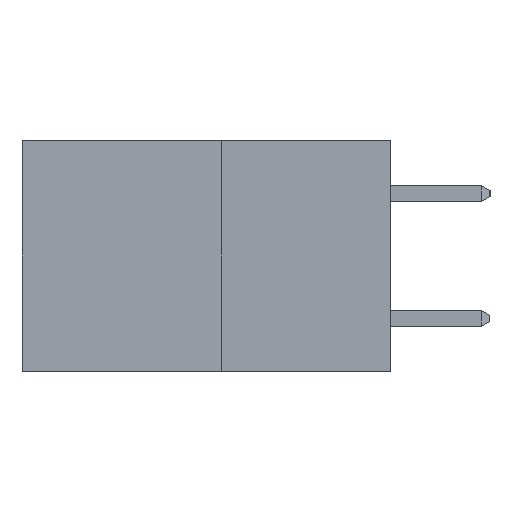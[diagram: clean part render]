
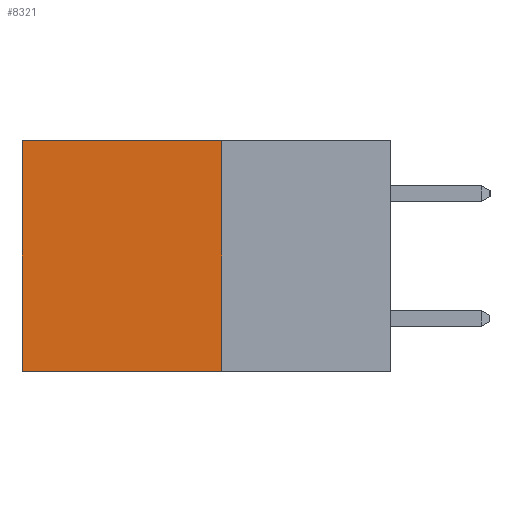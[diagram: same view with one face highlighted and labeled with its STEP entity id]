
A CAD part, left-side view. The second image highlights one B-rep face of the part: STEP entity #8321.
In plain terms, the highlighted planar face has unit normal (-1, 0, 0).
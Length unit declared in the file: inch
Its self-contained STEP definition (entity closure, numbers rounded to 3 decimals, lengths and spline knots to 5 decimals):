
#217 = VECTOR ( 'NONE', #8295, 39.37008 ) ;
#416 = VERTEX_POINT ( 'NONE', #7697 ) ;
#633 = CARTESIAN_POINT ( 'NONE',  ( 0.277, 0.59, -0.37 ) ) ;
#1566 = ORIENTED_EDGE ( 'NONE', *, *, #2854, .T. ) ;
#1673 = DIRECTION ( 'NONE',  ( 0., 0., -1. ) ) ;
#1694 = CARTESIAN_POINT ( 'NONE',  ( 0.277, 0.27, -0.37 ) ) ;
#1730 = VECTOR ( 'NONE', #4963, 39.37008 ) ;
#2251 = ORIENTED_EDGE ( 'NONE', *, *, #8538, .F. ) ;
#2705 = LINE ( 'NONE', #8316, #217 ) ;
#2854 = EDGE_CURVE ( 'NONE', #7122, #3989, #6411, .T. ) ;
#3082 = DIRECTION ( 'NONE',  ( 0., 0., -1. ) ) ;
#3104 = DIRECTION ( 'NONE',  ( 1., 0., 0. ) ) ;
#3123 = PLANE ( 'NONE',  #8015 ) ;
#3143 = ORIENTED_EDGE ( 'NONE', *, *, #5931, .F. ) ;
#3219 = CARTESIAN_POINT ( 'NONE',  ( 0.277, 0.27, -0.37 ) ) ;
#3271 = VERTEX_POINT ( 'NONE', #3448 ) ;
#3448 = CARTESIAN_POINT ( 'NONE',  ( 0.277, 0.27, 0. ) ) ;
#3715 = LINE ( 'NONE', #4950, #1730 ) ;
#3786 = CARTESIAN_POINT ( 'NONE',  ( 0.277, 0.59, 0. ) ) ;
#3989 = VERTEX_POINT ( 'NONE', #4318 ) ;
#4318 = CARTESIAN_POINT ( 'NONE',  ( 0.277, 0.59, -0.37 ) ) ;
#4448 = VECTOR ( 'NONE', #5295, 39.37008 ) ;
#4883 = EDGE_CURVE ( 'NONE', #3271, #7122, #2705, .T. ) ;
#4950 = CARTESIAN_POINT ( 'NONE',  ( 0.277, 0.27, -0.37 ) ) ;
#4963 = DIRECTION ( 'NONE',  ( 0., 1., 0. ) ) ;
#5289 = EDGE_LOOP ( 'NONE', ( #1566, #3143, #2251, #6467 ) ) ;
#5295 = DIRECTION ( 'NONE',  ( 0., 0., -1. ) ) ;
#5931 = EDGE_CURVE ( 'NONE', #416, #3989, #3715, .T. ) ;
#6310 = VECTOR ( 'NONE', #1673, 39.37008 ) ;
#6411 = LINE ( 'NONE', #633, #4448 ) ;
#6467 = ORIENTED_EDGE ( 'NONE', *, *, #4883, .T. ) ;
#6779 = LINE ( 'NONE', #1694, #6310 ) ;
#7122 = VERTEX_POINT ( 'NONE', #3786 ) ;
#7697 = CARTESIAN_POINT ( 'NONE',  ( 0.277, 0.27, -0.37 ) ) ;
#8015 = AXIS2_PLACEMENT_3D ( 'NONE', #3219, #3104, #3082 ) ;
#8173 = FACE_OUTER_BOUND ( 'NONE', #5289, .T. ) ;
#8295 = DIRECTION ( 'NONE',  ( 0., 1., 0. ) ) ;
#8316 = CARTESIAN_POINT ( 'NONE',  ( 0.277, 0.27, 0. ) ) ;
#8321 = ADVANCED_FACE ( 'NONE', ( #8173 ), #3123, .F. ) ;
#8538 = EDGE_CURVE ( 'NONE', #3271, #416, #6779, .T. ) ;
